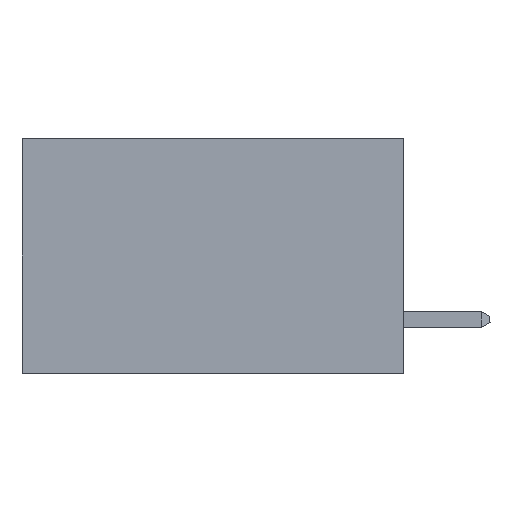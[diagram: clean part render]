
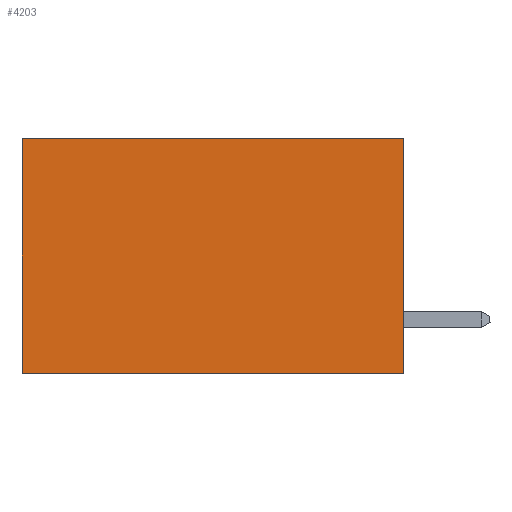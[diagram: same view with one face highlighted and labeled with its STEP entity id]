
A CAD part, left-side view. The second image highlights one B-rep face of the part: STEP entity #4203.
In plain terms, the highlighted planar face has unit normal (-1, 0, 0).
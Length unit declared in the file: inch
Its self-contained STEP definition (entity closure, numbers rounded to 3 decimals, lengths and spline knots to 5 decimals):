
#55 = DIRECTION ( 'NONE',  ( 0., 1., 0. ) ) ;
#1661 = DIRECTION ( 'NONE',  ( 0., 0., -1. ) ) ;
#1869 = VERTEX_POINT ( 'NONE', #11882 ) ;
#3073 = DIRECTION ( 'NONE',  ( 0., 0., -1. ) ) ;
#3135 = CARTESIAN_POINT ( 'NONE',  ( 0.2875, 0., -0.37 ) ) ;
#4114 = ORIENTED_EDGE ( 'NONE', *, *, #19921, .F. ) ;
#4203 = ADVANCED_FACE ( 'NONE', ( #9920 ), #7471, .F. ) ;
#5074 = CARTESIAN_POINT ( 'NONE',  ( 0.2875, 0., -0.37 ) ) ;
#5261 = CARTESIAN_POINT ( 'NONE',  ( 0.2875, 0.6, -0.37 ) ) ;
#5583 = LINE ( 'NONE', #10229, #15176 ) ;
#5799 = AXIS2_PLACEMENT_3D ( 'NONE', #19033, #13817, #5940 ) ;
#5940 = DIRECTION ( 'NONE',  ( 0., 0., -1. ) ) ;
#7120 = VECTOR ( 'NONE', #13172, 39.37008 ) ;
#7471 = PLANE ( 'NONE',  #5799 ) ;
#8924 = LINE ( 'NONE', #11739, #7120 ) ;
#8950 = EDGE_LOOP ( 'NONE', ( #15930, #17146, #4114, #16628 ) ) ;
#9776 = VECTOR ( 'NONE', #55, 39.37008 ) ;
#9826 = CARTESIAN_POINT ( 'NONE',  ( 0.2875, 0.6, 0. ) ) ;
#9920 = FACE_OUTER_BOUND ( 'NONE', #8950, .T. ) ;
#10229 = CARTESIAN_POINT ( 'NONE',  ( 0.2875, 0., 0. ) ) ;
#10698 = VERTEX_POINT ( 'NONE', #5261 ) ;
#11739 = CARTESIAN_POINT ( 'NONE',  ( 0.2875, 0., 0. ) ) ;
#11882 = CARTESIAN_POINT ( 'NONE',  ( 0.2875, 0., 0. ) ) ;
#12627 = LINE ( 'NONE', #5074, #9776 ) ;
#13172 = DIRECTION ( 'NONE',  ( 0., 1., 0. ) ) ;
#13817 = DIRECTION ( 'NONE',  ( 1., 0., 0. ) ) ;
#13998 = EDGE_CURVE ( 'NONE', #20302, #10698, #12627, .T. ) ;
#15176 = VECTOR ( 'NONE', #1661, 39.37008 ) ;
#15930 = ORIENTED_EDGE ( 'NONE', *, *, #18912, .T. ) ;
#16208 = CARTESIAN_POINT ( 'NONE',  ( 0.2875, 0.6, 0. ) ) ;
#16528 = VECTOR ( 'NONE', #3073, 39.37008 ) ;
#16628 = ORIENTED_EDGE ( 'NONE', *, *, #20487, .T. ) ;
#17146 = ORIENTED_EDGE ( 'NONE', *, *, #13998, .F. ) ;
#18912 = EDGE_CURVE ( 'NONE', #20906, #10698, #20972, .T. ) ;
#19033 = CARTESIAN_POINT ( 'NONE',  ( 0.2875, 0., 0. ) ) ;
#19921 = EDGE_CURVE ( 'NONE', #1869, #20302, #5583, .T. ) ;
#20302 = VERTEX_POINT ( 'NONE', #3135 ) ;
#20487 = EDGE_CURVE ( 'NONE', #1869, #20906, #8924, .T. ) ;
#20906 = VERTEX_POINT ( 'NONE', #9826 ) ;
#20972 = LINE ( 'NONE', #16208, #16528 ) ;
